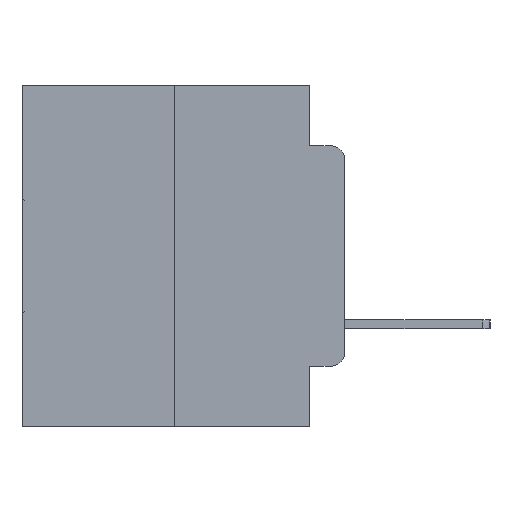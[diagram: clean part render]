
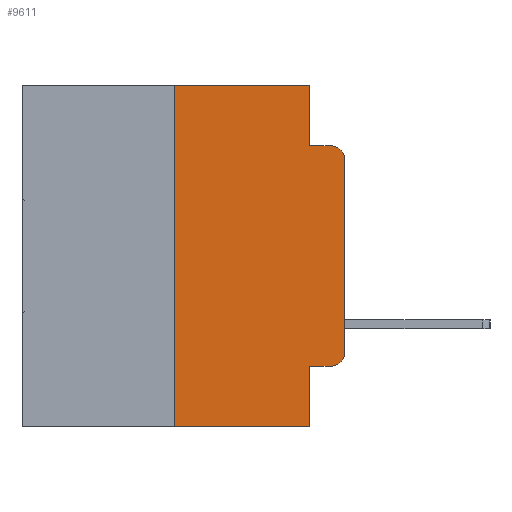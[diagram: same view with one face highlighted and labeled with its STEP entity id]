
A CAD part, left-side view. The second image highlights one B-rep face of the part: STEP entity #9611.
In plain terms, the highlighted planar face has unit normal (-1, 0, 0).
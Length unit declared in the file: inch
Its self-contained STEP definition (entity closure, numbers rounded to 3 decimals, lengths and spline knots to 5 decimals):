
#761 = EDGE_CURVE ( 'NONE', #26936, #11218, #21577, .T. ) ;
#804 = CARTESIAN_POINT ( 'NONE',  ( 0., 0.02, -0.4115 ) ) ;
#906 = EDGE_CURVE ( 'NONE', #12471, #3351, #24833, .T. ) ;
#1572 = LINE ( 'NONE', #3177, #12769 ) ;
#2218 = EDGE_CURVE ( 'NONE', #17604, #26936, #1572, .T. ) ;
#2300 = VECTOR ( 'NONE', #17099, 39.37008 ) ;
#2307 = VECTOR ( 'NONE', #11450, 39.37008 ) ;
#2404 = VECTOR ( 'NONE', #10619, 39.37008 ) ;
#2475 = CARTESIAN_POINT ( 'NONE',  ( 0., 0.25, 0. ) ) ;
#2783 = ORIENTED_EDGE ( 'NONE', *, *, #906, .T. ) ;
#3177 = CARTESIAN_POINT ( 'NONE',  ( 0., 0.25, 0. ) ) ;
#3210 = CARTESIAN_POINT ( 'NONE',  ( 0., 0., -0.3915 ) ) ;
#3351 = VERTEX_POINT ( 'NONE', #25350 ) ;
#3667 = EDGE_CURVE ( 'NONE', #17416, #18540, #4432, .T. ) ;
#4221 = VECTOR ( 'NONE', #16380, 39.37008 ) ;
#4432 = LINE ( 'NONE', #18261, #9549 ) ;
#4676 = ORIENTED_EDGE ( 'NONE', *, *, #21376, .T. ) ;
#5163 = EDGE_LOOP ( 'NONE', ( #2783, #17026, #15533, #19814, #23662, #12630, #25479, #7139, #18997, #4676 ) ) ;
#5588 = VECTOR ( 'NONE', #23897, 39.37008 ) ;
#5840 = CARTESIAN_POINT ( 'NONE',  ( 0., 0.051, 0. ) ) ;
#7139 = ORIENTED_EDGE ( 'NONE', *, *, #26287, .F. ) ;
#7170 = PLANE ( 'NONE',  #24723 ) ;
#8380 = DIRECTION ( 'NONE',  ( -1., 0., 0. ) ) ;
#8387 = VERTEX_POINT ( 'NONE', #11681 ) ;
#8414 = CARTESIAN_POINT ( 'NONE',  ( 0., 0.051, 0. ) ) ;
#9549 = VECTOR ( 'NONE', #16087, 39.37008 ) ;
#9611 = ADVANCED_FACE ( 'NONE', ( #17548 ), #7170, .F. ) ;
#10619 = DIRECTION ( 'NONE',  ( 0., 0., -1. ) ) ;
#10692 = CARTESIAN_POINT ( 'NONE',  ( 0., 0.25, -0.5 ) ) ;
#10974 = AXIS2_PLACEMENT_3D ( 'NONE', #21419, #8380, #23528 ) ;
#11218 = VERTEX_POINT ( 'NONE', #5840 ) ;
#11450 = DIRECTION ( 'NONE',  ( 0., 0., 1. ) ) ;
#11681 = CARTESIAN_POINT ( 'NONE',  ( 0., 0.051, -0.4115 ) ) ;
#11996 = CARTESIAN_POINT ( 'NONE',  ( 0., 0.473, 0. ) ) ;
#12146 = DIRECTION ( 'NONE',  ( -1., 0., 0. ) ) ;
#12471 = VERTEX_POINT ( 'NONE', #3210 ) ;
#12630 = ORIENTED_EDGE ( 'NONE', *, *, #2218, .F. ) ;
#12769 = VECTOR ( 'NONE', #26511, 39.37008 ) ;
#12800 = AXIS2_PLACEMENT_3D ( 'NONE', #25025, #12146, #27144 ) ;
#13851 = DIRECTION ( 'NONE',  ( 0., 0., -1. ) ) ;
#14812 = LINE ( 'NONE', #27686, #2300 ) ;
#15488 = VERTEX_POINT ( 'NONE', #804 ) ;
#15533 = ORIENTED_EDGE ( 'NONE', *, *, #3667, .F. ) ;
#15766 = CIRCLE ( 'NONE', #10974, 0.02 ) ;
#16087 = DIRECTION ( 'NONE',  ( 0., -1., 0. ) ) ;
#16380 = DIRECTION ( 'NONE',  ( 0., -1., 0. ) ) ;
#16657 = CARTESIAN_POINT ( 'NONE',  ( 0., 0., 0. ) ) ;
#16877 = VERTEX_POINT ( 'NONE', #27069 ) ;
#17026 = ORIENTED_EDGE ( 'NONE', *, *, #19219, .T. ) ;
#17099 = DIRECTION ( 'NONE',  ( 0., -1., 0. ) ) ;
#17416 = VERTEX_POINT ( 'NONE', #18817 ) ;
#17548 = FACE_OUTER_BOUND ( 'NONE', #5163, .T. ) ;
#17604 = VERTEX_POINT ( 'NONE', #10692 ) ;
#18261 = CARTESIAN_POINT ( 'NONE',  ( 0., 0.051, -0.0885 ) ) ;
#18540 = VERTEX_POINT ( 'NONE', #24672 ) ;
#18646 = CARTESIAN_POINT ( 'NONE',  ( 0., 0.051, 0. ) ) ;
#18817 = CARTESIAN_POINT ( 'NONE',  ( 0., 0.051, -0.0885 ) ) ;
#18997 = ORIENTED_EDGE ( 'NONE', *, *, #20667, .T. ) ;
#19219 = EDGE_CURVE ( 'NONE', #3351, #18540, #28113, .T. ) ;
#19629 = CARTESIAN_POINT ( 'NONE',  ( 0., 0.473, -0.5 ) ) ;
#19814 = ORIENTED_EDGE ( 'NONE', *, *, #27250, .F. ) ;
#19938 = LINE ( 'NONE', #8414, #2404 ) ;
#20667 = EDGE_CURVE ( 'NONE', #8387, #15488, #14812, .T. ) ;
#20801 = EDGE_CURVE ( 'NONE', #17604, #16877, #27786, .T. ) ;
#21376 = EDGE_CURVE ( 'NONE', #15488, #12471, #15766, .T. ) ;
#21419 = CARTESIAN_POINT ( 'NONE',  ( 0., 0.02, -0.3915 ) ) ;
#21577 = LINE ( 'NONE', #11996, #4221 ) ;
#21724 = VECTOR ( 'NONE', #27158, 39.37008 ) ;
#22438 = CARTESIAN_POINT ( 'NONE',  ( 0., 0.473, 0. ) ) ;
#23528 = DIRECTION ( 'NONE',  ( 0., 0., -1. ) ) ;
#23662 = ORIENTED_EDGE ( 'NONE', *, *, #761, .F. ) ;
#23897 = DIRECTION ( 'NONE',  ( 0., -1., 0. ) ) ;
#24672 = CARTESIAN_POINT ( 'NONE',  ( 0., 0.02, -0.0885 ) ) ;
#24723 = AXIS2_PLACEMENT_3D ( 'NONE', #22438, #26640, #13851 ) ;
#24833 = LINE ( 'NONE', #16657, #2307 ) ;
#25025 = CARTESIAN_POINT ( 'NONE',  ( 0., 0.02, -0.1085 ) ) ;
#25350 = CARTESIAN_POINT ( 'NONE',  ( 0., 0., -0.1085 ) ) ;
#25479 = ORIENTED_EDGE ( 'NONE', *, *, #20801, .T. ) ;
#26287 = EDGE_CURVE ( 'NONE', #8387, #16877, #19938, .T. ) ;
#26511 = DIRECTION ( 'NONE',  ( 0., 0., 1. ) ) ;
#26640 = DIRECTION ( 'NONE',  ( 1., 0., 0. ) ) ;
#26936 = VERTEX_POINT ( 'NONE', #2475 ) ;
#27069 = CARTESIAN_POINT ( 'NONE',  ( 0., 0.051, -0.5 ) ) ;
#27144 = DIRECTION ( 'NONE',  ( 0., 0., -1. ) ) ;
#27158 = DIRECTION ( 'NONE',  ( 0., 0., -1. ) ) ;
#27250 = EDGE_CURVE ( 'NONE', #11218, #17416, #27312, .T. ) ;
#27312 = LINE ( 'NONE', #18646, #21724 ) ;
#27686 = CARTESIAN_POINT ( 'NONE',  ( 0., 0.051, -0.4115 ) ) ;
#27786 = LINE ( 'NONE', #19629, #5588 ) ;
#28113 = CIRCLE ( 'NONE', #12800, 0.02 ) ;
